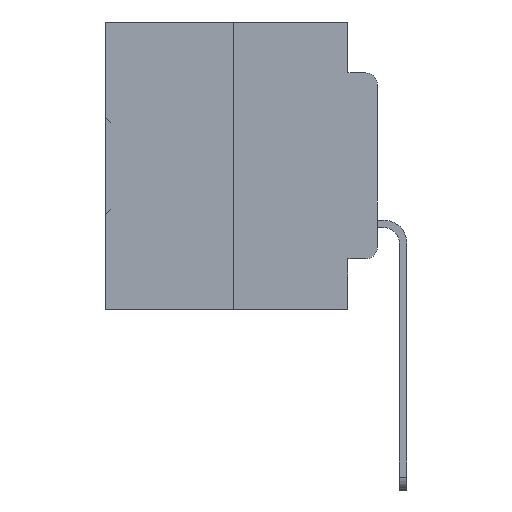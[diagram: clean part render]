
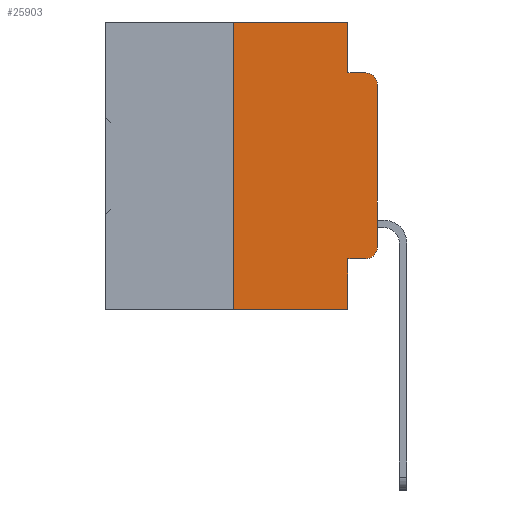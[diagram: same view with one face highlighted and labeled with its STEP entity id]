
A CAD part, left-side view. The second image highlights one B-rep face of the part: STEP entity #25903.
In plain terms, the highlighted planar face has unit normal (-1, 0, 0).
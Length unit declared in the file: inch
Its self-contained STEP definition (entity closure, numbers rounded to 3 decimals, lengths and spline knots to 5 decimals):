
#112 = AXIS2_PLACEMENT_3D ( 'NONE', #29053, #12275, #31850 ) ;
#357 = DIRECTION ( 'NONE',  ( 0., 0., 1. ) ) ;
#365 = VECTOR ( 'NONE', #15510, 39.37008 ) ;
#615 = VERTEX_POINT ( 'NONE', #28097 ) ;
#732 = CARTESIAN_POINT ( 'NONE',  ( 0., 0.051, -0.5 ) ) ;
#1177 = VERTEX_POINT ( 'NONE', #8321 ) ;
#1210 = LINE ( 'NONE', #33758, #15656 ) ;
#2261 = LINE ( 'NONE', #28834, #22340 ) ;
#2456 = VECTOR ( 'NONE', #33498, 39.37008 ) ;
#3224 = DIRECTION ( 'NONE',  ( 1., 0., 0. ) ) ;
#3558 = AXIS2_PLACEMENT_3D ( 'NONE', #14958, #34516, #17774 ) ;
#3935 = LINE ( 'NONE', #30747, #10768 ) ;
#4102 = LINE ( 'NONE', #11567, #31503 ) ;
#4106 = VERTEX_POINT ( 'NONE', #13245 ) ;
#5448 = DIRECTION ( 'NONE',  ( 0., 0., -1. ) ) ;
#7225 = ORIENTED_EDGE ( 'NONE', *, *, #34294, .T. ) ;
#7353 = FACE_OUTER_BOUND ( 'NONE', #16055, .T. ) ;
#8321 = CARTESIAN_POINT ( 'NONE',  ( 0., 0.051, -0.4115 ) ) ;
#8458 = VERTEX_POINT ( 'NONE', #29253 ) ;
#9023 = VERTEX_POINT ( 'NONE', #23360 ) ;
#9071 = LINE ( 'NONE', #11047, #365 ) ;
#9976 = CARTESIAN_POINT ( 'NONE',  ( 0., 0.051, 0. ) ) ;
#10550 = CIRCLE ( 'NONE', #112, 0.02 ) ;
#10768 = VECTOR ( 'NONE', #5448, 39.37008 ) ;
#11047 = CARTESIAN_POINT ( 'NONE',  ( 0., 0., 0. ) ) ;
#11080 = EDGE_CURVE ( 'NONE', #1177, #36478, #3935, .T. ) ;
#11567 = CARTESIAN_POINT ( 'NONE',  ( 0., 0.051, -0.4115 ) ) ;
#11680 = ORIENTED_EDGE ( 'NONE', *, *, #12702, .T. ) ;
#12275 = DIRECTION ( 'NONE',  ( -1., 0., 0. ) ) ;
#12702 = EDGE_CURVE ( 'NONE', #615, #36478, #23404, .T. ) ;
#13162 = EDGE_CURVE ( 'NONE', #9023, #27498, #36413, .T. ) ;
#13245 = CARTESIAN_POINT ( 'NONE',  ( 0., 0., -0.3915 ) ) ;
#13597 = VECTOR ( 'NONE', #26772, 39.37008 ) ;
#13663 = CARTESIAN_POINT ( 'NONE',  ( 0., 0.473, 0. ) ) ;
#14518 = DIRECTION ( 'NONE',  ( 0., -1., 0. ) ) ;
#14958 = CARTESIAN_POINT ( 'NONE',  ( 0., 0.02, -0.1085 ) ) ;
#15377 = LINE ( 'NONE', #9976, #13597 ) ;
#15510 = DIRECTION ( 'NONE',  ( 0., 0., 1. ) ) ;
#15656 = VECTOR ( 'NONE', #36526, 39.37008 ) ;
#16055 = EDGE_LOOP ( 'NONE', ( #31365, #35735, #26130, #19583, #16532, #33157, #11680, #36607, #7225, #25323 ) ) ;
#16532 = ORIENTED_EDGE ( 'NONE', *, *, #13162, .F. ) ;
#16757 = CARTESIAN_POINT ( 'NONE',  ( 0., 0.473, -0.5 ) ) ;
#17774 = DIRECTION ( 'NONE',  ( 0., 0., -1. ) ) ;
#19317 = EDGE_CURVE ( 'NONE', #27851, #4106, #10550, .T. ) ;
#19583 = ORIENTED_EDGE ( 'NONE', *, *, #26099, .F. ) ;
#20166 = CARTESIAN_POINT ( 'NONE',  ( 0., 0.02, -0.0885 ) ) ;
#20494 = EDGE_CURVE ( 'NONE', #615, #9023, #2261, .T. ) ;
#21035 = VERTEX_POINT ( 'NONE', #29882 ) ;
#21602 = VECTOR ( 'NONE', #33350, 39.37008 ) ;
#22340 = VECTOR ( 'NONE', #357, 39.37008 ) ;
#23145 = DIRECTION ( 'NONE',  ( 0., 0., -1. ) ) ;
#23360 = CARTESIAN_POINT ( 'NONE',  ( 0., 0.25, 0. ) ) ;
#23404 = LINE ( 'NONE', #16757, #2456 ) ;
#23688 = CIRCLE ( 'NONE', #3558, 0.02 ) ;
#23842 = AXIS2_PLACEMENT_3D ( 'NONE', #25810, #3224, #23145 ) ;
#25323 = ORIENTED_EDGE ( 'NONE', *, *, #19317, .T. ) ;
#25396 = EDGE_CURVE ( 'NONE', #8458, #36345, #23688, .T. ) ;
#25810 = CARTESIAN_POINT ( 'NONE',  ( 0., 0.473, 0. ) ) ;
#25903 = ADVANCED_FACE ( 'NONE', ( #7353 ), #28625, .F. ) ;
#26099 = EDGE_CURVE ( 'NONE', #27498, #21035, #15377, .T. ) ;
#26130 = ORIENTED_EDGE ( 'NONE', *, *, #27981, .F. ) ;
#26772 = DIRECTION ( 'NONE',  ( 0., 0., -1. ) ) ;
#27498 = VERTEX_POINT ( 'NONE', #31722 ) ;
#27851 = VERTEX_POINT ( 'NONE', #33169 ) ;
#27981 = EDGE_CURVE ( 'NONE', #21035, #36345, #1210, .T. ) ;
#28097 = CARTESIAN_POINT ( 'NONE',  ( 0., 0.25, -0.5 ) ) ;
#28625 = PLANE ( 'NONE',  #23842 ) ;
#28834 = CARTESIAN_POINT ( 'NONE',  ( 0., 0.25, 0. ) ) ;
#29053 = CARTESIAN_POINT ( 'NONE',  ( 0., 0.02, -0.3915 ) ) ;
#29253 = CARTESIAN_POINT ( 'NONE',  ( 0., 0., -0.1085 ) ) ;
#29882 = CARTESIAN_POINT ( 'NONE',  ( 0., 0.051, -0.0885 ) ) ;
#30747 = CARTESIAN_POINT ( 'NONE',  ( 0., 0.051, 0. ) ) ;
#31365 = ORIENTED_EDGE ( 'NONE', *, *, #34781, .T. ) ;
#31503 = VECTOR ( 'NONE', #14518, 39.37008 ) ;
#31722 = CARTESIAN_POINT ( 'NONE',  ( 0., 0.051, 0. ) ) ;
#31850 = DIRECTION ( 'NONE',  ( 0., 0., -1. ) ) ;
#33157 = ORIENTED_EDGE ( 'NONE', *, *, #20494, .F. ) ;
#33169 = CARTESIAN_POINT ( 'NONE',  ( 0., 0.02, -0.4115 ) ) ;
#33350 = DIRECTION ( 'NONE',  ( 0., -1., 0. ) ) ;
#33498 = DIRECTION ( 'NONE',  ( 0., -1., 0. ) ) ;
#33758 = CARTESIAN_POINT ( 'NONE',  ( 0., 0.051, -0.0885 ) ) ;
#34294 = EDGE_CURVE ( 'NONE', #1177, #27851, #4102, .T. ) ;
#34516 = DIRECTION ( 'NONE',  ( -1., 0., 0. ) ) ;
#34781 = EDGE_CURVE ( 'NONE', #4106, #8458, #9071, .T. ) ;
#35735 = ORIENTED_EDGE ( 'NONE', *, *, #25396, .T. ) ;
#36345 = VERTEX_POINT ( 'NONE', #20166 ) ;
#36413 = LINE ( 'NONE', #13663, #21602 ) ;
#36478 = VERTEX_POINT ( 'NONE', #732 ) ;
#36526 = DIRECTION ( 'NONE',  ( 0., -1., 0. ) ) ;
#36607 = ORIENTED_EDGE ( 'NONE', *, *, #11080, .F. ) ;
